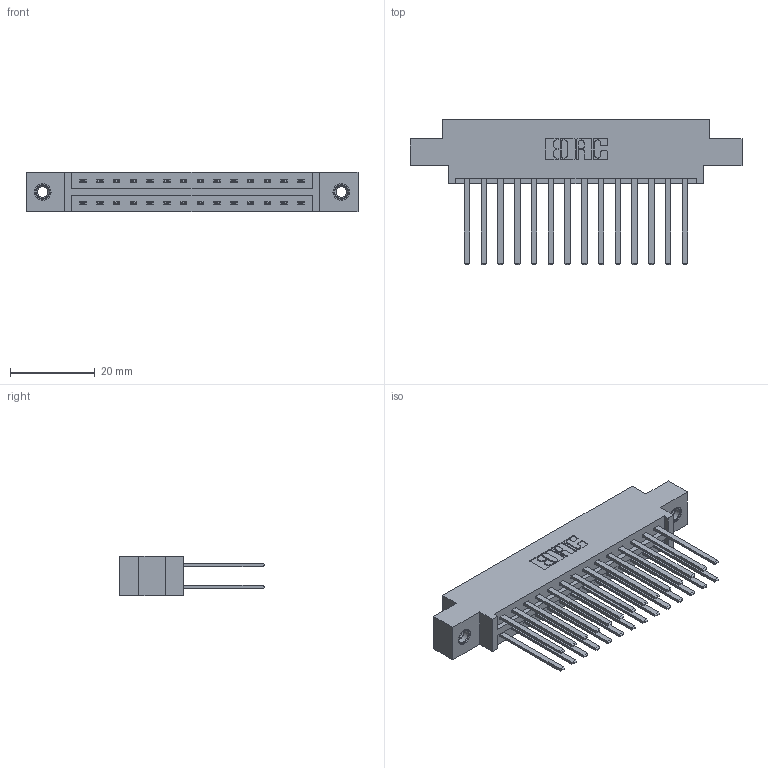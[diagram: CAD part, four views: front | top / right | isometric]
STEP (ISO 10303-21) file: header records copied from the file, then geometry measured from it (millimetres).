
FILE_DESCRIPTION (( 'STEP AP203' ), '1' );
FILE_NAME ('387-028-544-807.STEP', '2019-10-16T22:32:28', ( '' ), ( '' ), 'SwSTEP 2.0', 'SolidWorks 2016', '' );
FILE_SCHEMA (( 'CONFIG_CONTROL_DESIGN' ));
Length unit declared in the file: inch
Products named in the file (4): 387-028-544-807; 345-292-001_345-293-144; 345-250-001_345-250-005-103; 337 Part_0.170 Offset - 0.156 Dia-TI
Assembly tree (31 placements, depth 2):
  387-028-544-807
    337 Part_0.170 Offset - 0.156 Dia-TI
    345-292-001_345-293-144  x28
    345-250-001_345-250-005-103  x2
Bounding box: 78.49 x 34.3 x 9.4 mm (x, y, z)
Volume: 8160.3 mm3; surface area: 10379.2 mm2
Topology: 31 solids, 31 shells, 1522 faces, 4463 edges, 2930 vertices
Faces by surface type: plane 1058, cylinder 448, cone 12, torus 4
Entity records: 15610 total; most frequent: CARTESIAN_POINT 2633, ORIENTED_EDGE 2562, DIRECTION 2319, EDGE_CURVE 1281, VECTOR 1137, LINE 1137, VERTEX_POINT 848, AXIS2_PLACEMENT_3D 591
